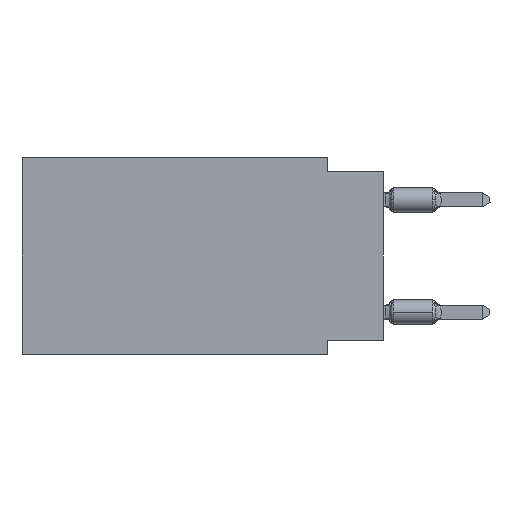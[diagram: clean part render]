
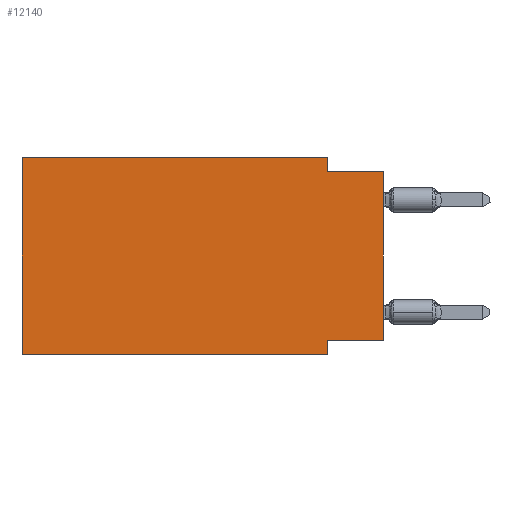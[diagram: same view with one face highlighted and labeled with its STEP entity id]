
A CAD part, left-side view. The second image highlights one B-rep face of the part: STEP entity #12140.
In plain terms, the highlighted planar face has unit normal (-1, 0, 0).
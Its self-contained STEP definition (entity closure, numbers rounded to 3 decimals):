
#130 = EDGE_CURVE ( 'NONE', #36394, #3868, #45524, .T. ) ;
#348 = VECTOR ( 'NONE', #11020, 1000. ) ;
#618 = CARTESIAN_POINT ( 'NONE',  ( 0., 0., -8.255 ) ) ;
#1778 = LINE ( 'NONE', #34018, #30842 ) ;
#2932 = LINE ( 'NONE', #17707, #348 ) ;
#3604 = CARTESIAN_POINT ( 'NONE',  ( 0., 2.54, 0. ) ) ;
#3629 = VERTEX_POINT ( 'NONE', #16886 ) ;
#3868 = VERTEX_POINT ( 'NONE', #5784 ) ;
#5350 = DIRECTION ( 'NONE',  ( 0., 0., -1. ) ) ;
#5456 = ORIENTED_EDGE ( 'NONE', *, *, #39271, .F. ) ;
#5751 = CARTESIAN_POINT ( 'NONE',  ( 0., 16.383, -8.89 ) ) ;
#5784 = CARTESIAN_POINT ( 'NONE',  ( 0., 2.54, -8.89 ) ) ;
#6148 = PLANE ( 'NONE',  #28745 ) ;
#6812 = CARTESIAN_POINT ( 'NONE',  ( 0., 2.54, -8.255 ) ) ;
#7114 = CARTESIAN_POINT ( 'NONE',  ( 0., 0., -0.635 ) ) ;
#9464 = EDGE_CURVE ( 'NONE', #30376, #42415, #43792, .T. ) ;
#9630 = FACE_OUTER_BOUND ( 'NONE', #14398, .T. ) ;
#9845 = DIRECTION ( 'NONE',  ( 1., 0., 0. ) ) ;
#11020 = DIRECTION ( 'NONE',  ( 0., -1., 0. ) ) ;
#11461 = DIRECTION ( 'NONE',  ( 0., 1., 0. ) ) ;
#11842 = ORIENTED_EDGE ( 'NONE', *, *, #29599, .F. ) ;
#12023 = CARTESIAN_POINT ( 'NONE',  ( 0., 0., -0.635 ) ) ;
#12140 = ADVANCED_FACE ( 'NONE', ( #9630 ), #6148, .F. ) ;
#13446 = LINE ( 'NONE', #27492, #36661 ) ;
#14398 = EDGE_LOOP ( 'NONE', ( #19487, #39351, #5456, #11842, #45232, #32725, #43994, #35334 ) ) ;
#14876 = LINE ( 'NONE', #43640, #31374 ) ;
#16886 = CARTESIAN_POINT ( 'NONE',  ( 0., 16.383, 0. ) ) ;
#17707 = CARTESIAN_POINT ( 'NONE',  ( 0., 16.383, 0. ) ) ;
#18523 = VERTEX_POINT ( 'NONE', #6812 ) ;
#18671 = VERTEX_POINT ( 'NONE', #3604 ) ;
#19487 = ORIENTED_EDGE ( 'NONE', *, *, #43861, .T. ) ;
#19546 = DIRECTION ( 'NONE',  ( 0., 0., 1. ) ) ;
#21357 = DIRECTION ( 'NONE',  ( 0., -1., 0. ) ) ;
#21995 = CARTESIAN_POINT ( 'NONE',  ( 0., 2.54, -8.89 ) ) ;
#22918 = DIRECTION ( 'NONE',  ( 0., 0., 1. ) ) ;
#23308 = VECTOR ( 'NONE', #5350, 1000. ) ;
#23677 = DIRECTION ( 'NONE',  ( 0., 0., -1. ) ) ;
#24727 = EDGE_CURVE ( 'NONE', #36394, #3629, #14876, .T. ) ;
#26595 = VECTOR ( 'NONE', #21357, 1000. ) ;
#27492 = CARTESIAN_POINT ( 'NONE',  ( 0., 2.54, 0. ) ) ;
#28019 = CARTESIAN_POINT ( 'NONE',  ( 0., 16.383, -8.89 ) ) ;
#28745 = AXIS2_PLACEMENT_3D ( 'NONE', #30808, #9845, #23677 ) ;
#29599 = EDGE_CURVE ( 'NONE', #3629, #18671, #2932, .T. ) ;
#30194 = VECTOR ( 'NONE', #11461, 1000. ) ;
#30376 = VERTEX_POINT ( 'NONE', #37949 ) ;
#30808 = CARTESIAN_POINT ( 'NONE',  ( 0., 16.383, 0. ) ) ;
#30842 = VECTOR ( 'NONE', #19546, 1000. ) ;
#31374 = VECTOR ( 'NONE', #22918, 1000. ) ;
#32725 = ORIENTED_EDGE ( 'NONE', *, *, #130, .T. ) ;
#34018 = CARTESIAN_POINT ( 'NONE',  ( 0., 0., 0. ) ) ;
#35116 = VERTEX_POINT ( 'NONE', #44205 ) ;
#35334 = ORIENTED_EDGE ( 'NONE', *, *, #45457, .F. ) ;
#35946 = VECTOR ( 'NONE', #40127, 1000. ) ;
#36309 = LINE ( 'NONE', #618, #30194 ) ;
#36394 = VERTEX_POINT ( 'NONE', #5751 ) ;
#36661 = VECTOR ( 'NONE', #41532, 1000. ) ;
#37534 = EDGE_CURVE ( 'NONE', #18523, #3868, #39930, .T. ) ;
#37949 = CARTESIAN_POINT ( 'NONE',  ( 0., 2.54, -0.635 ) ) ;
#39271 = EDGE_CURVE ( 'NONE', #18671, #30376, #13446, .T. ) ;
#39351 = ORIENTED_EDGE ( 'NONE', *, *, #9464, .F. ) ;
#39930 = LINE ( 'NONE', #21995, #23308 ) ;
#40127 = DIRECTION ( 'NONE',  ( 0., -1., 0. ) ) ;
#41532 = DIRECTION ( 'NONE',  ( 0., 0., -1. ) ) ;
#42415 = VERTEX_POINT ( 'NONE', #7114 ) ;
#43640 = CARTESIAN_POINT ( 'NONE',  ( 0., 16.383, 0. ) ) ;
#43792 = LINE ( 'NONE', #12023, #35946 ) ;
#43861 = EDGE_CURVE ( 'NONE', #35116, #42415, #1778, .T. ) ;
#43994 = ORIENTED_EDGE ( 'NONE', *, *, #37534, .F. ) ;
#44205 = CARTESIAN_POINT ( 'NONE',  ( 0., 0., -8.255 ) ) ;
#45232 = ORIENTED_EDGE ( 'NONE', *, *, #24727, .F. ) ;
#45457 = EDGE_CURVE ( 'NONE', #35116, #18523, #36309, .T. ) ;
#45524 = LINE ( 'NONE', #28019, #26595 ) ;
